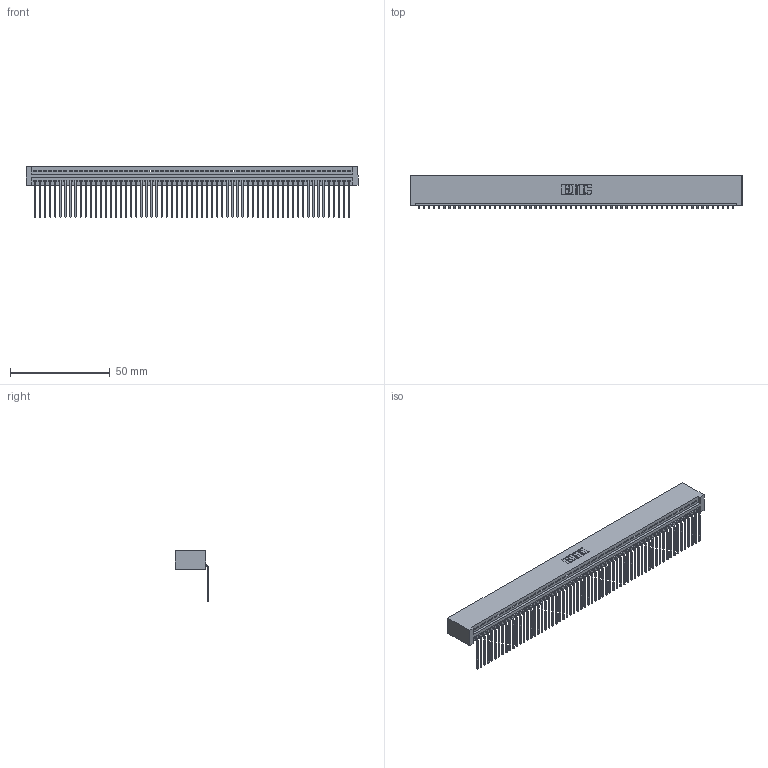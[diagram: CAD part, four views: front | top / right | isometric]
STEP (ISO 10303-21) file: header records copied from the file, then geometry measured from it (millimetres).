
FILE_DESCRIPTION (( 'STEP AP203' ), '1' );
FILE_NAME ('345-063-559-101.STEP', '2018-09-28T02:51:29', ( '' ), ( '' ), 'SwSTEP 2.0', 'SolidWorks 2016', '' );
FILE_SCHEMA (( 'CONFIG_CONTROL_DESIGN' ));
Length unit declared in the file: inch
Products named in the file (3): 345-292-001_558 559 Tail - 1; 345 Part_No Mounting Lugs; 345-063-559-101
Assembly tree (64 placements, depth 2):
  345-063-559-101
    345 Part_No Mounting Lugs
    345-292-001_558 559 Tail - 1  x63
Bounding box: 166.62 x 16.75 x 25.53 mm (x, y, z)
Volume: 16792.4 mm3; surface area: 24024.5 mm2
Topology: 64 solids, 64 shells, 3898 faces, 11783 edges, 7770 vertices
Faces by surface type: plane 2722, cylinder 1176
Entity records: 44395 total; most frequent: CARTESIAN_POINT 7697, ORIENTED_EDGE 7694, DIRECTION 6685, EDGE_CURVE 3847, LINE 3471, VECTOR 3471, VERTEX_POINT 2562, AXIS2_PLACEMENT_3D 1607
